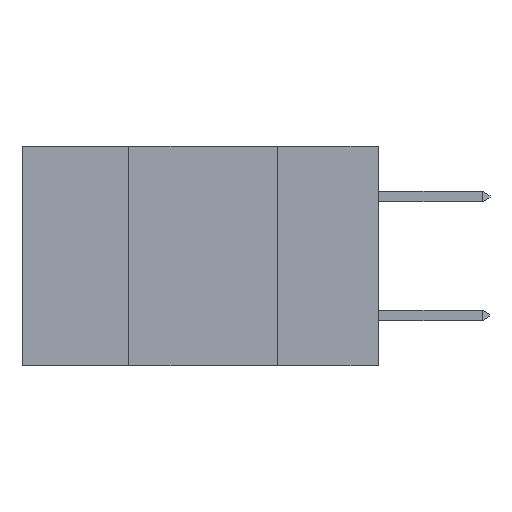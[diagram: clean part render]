
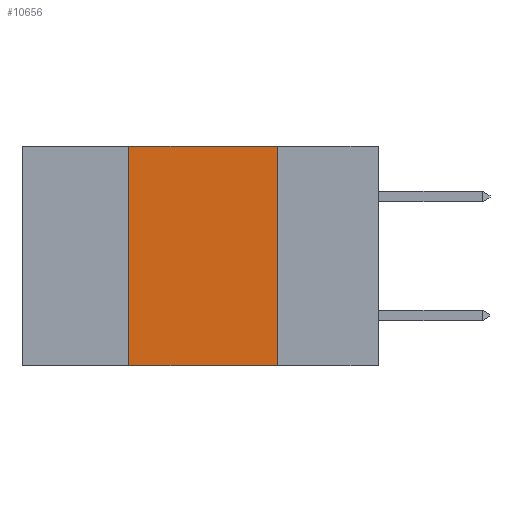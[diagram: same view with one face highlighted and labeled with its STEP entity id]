
A CAD part, left-side view. The second image highlights one B-rep face of the part: STEP entity #10656.
In plain terms, the highlighted planar face has unit normal (-1, 0, 0).
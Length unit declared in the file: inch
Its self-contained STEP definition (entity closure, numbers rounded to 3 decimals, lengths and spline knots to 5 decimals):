
#294 = ORIENTED_EDGE ( 'NONE', *, *, #7174, .F. ) ;
#372 = CARTESIAN_POINT ( 'NONE',  ( 0., 0.6, 0. ) ) ;
#556 = FACE_OUTER_BOUND ( 'NONE', #6729, .T. ) ;
#820 = CARTESIAN_POINT ( 'NONE',  ( 0., 0.42, 0. ) ) ;
#1115 = LINE ( 'NONE', #1299, #3602 ) ;
#1299 = CARTESIAN_POINT ( 'NONE',  ( 0., 0.17, 0. ) ) ;
#1372 = DIRECTION ( 'NONE',  ( 1., 0., 0. ) ) ;
#1731 = VERTEX_POINT ( 'NONE', #8355 ) ;
#2010 = LINE ( 'NONE', #10041, #11379 ) ;
#2060 = EDGE_CURVE ( 'NONE', #11722, #1731, #5029, .T. ) ;
#2134 = LINE ( 'NONE', #820, #2426 ) ;
#2426 = VECTOR ( 'NONE', #7510, 39.37008 ) ;
#3432 = DIRECTION ( 'NONE',  ( 0., -1., 0. ) ) ;
#3523 = AXIS2_PLACEMENT_3D ( 'NONE', #372, #1372, #8022 ) ;
#3602 = VECTOR ( 'NONE', #6457, 39.37008 ) ;
#4673 = ORIENTED_EDGE ( 'NONE', *, *, #8417, .F. ) ;
#5029 = LINE ( 'NONE', #8121, #9752 ) ;
#5770 = DIRECTION ( 'NONE',  ( 0., -1., 0. ) ) ;
#6155 = PLANE ( 'NONE',  #3523 ) ;
#6457 = DIRECTION ( 'NONE',  ( 0., 0., -1. ) ) ;
#6729 = EDGE_LOOP ( 'NONE', ( #294, #7328, #4673, #7801 ) ) ;
#6896 = CARTESIAN_POINT ( 'NONE',  ( 0., 0.42, -0.37 ) ) ;
#7108 = EDGE_CURVE ( 'NONE', #10996, #7354, #2010, .T. ) ;
#7174 = EDGE_CURVE ( 'NONE', #7354, #1731, #1115, .T. ) ;
#7328 = ORIENTED_EDGE ( 'NONE', *, *, #7108, .F. ) ;
#7354 = VERTEX_POINT ( 'NONE', #11519 ) ;
#7510 = DIRECTION ( 'NONE',  ( 0., 0., 1. ) ) ;
#7801 = ORIENTED_EDGE ( 'NONE', *, *, #2060, .T. ) ;
#8022 = DIRECTION ( 'NONE',  ( 0., 0., -1. ) ) ;
#8121 = CARTESIAN_POINT ( 'NONE',  ( 0., 0.6, -0.37 ) ) ;
#8355 = CARTESIAN_POINT ( 'NONE',  ( 0., 0.17, -0.37 ) ) ;
#8417 = EDGE_CURVE ( 'NONE', #11722, #10996, #2134, .T. ) ;
#9752 = VECTOR ( 'NONE', #3432, 39.37008 ) ;
#10041 = CARTESIAN_POINT ( 'NONE',  ( 0., 0.6, 0. ) ) ;
#10656 = ADVANCED_FACE ( 'NONE', ( #556 ), #6155, .F. ) ;
#10996 = VERTEX_POINT ( 'NONE', #12082 ) ;
#11379 = VECTOR ( 'NONE', #5770, 39.37008 ) ;
#11519 = CARTESIAN_POINT ( 'NONE',  ( 0., 0.17, 0. ) ) ;
#11722 = VERTEX_POINT ( 'NONE', #6896 ) ;
#12082 = CARTESIAN_POINT ( 'NONE',  ( 0., 0.42, 0. ) ) ;
